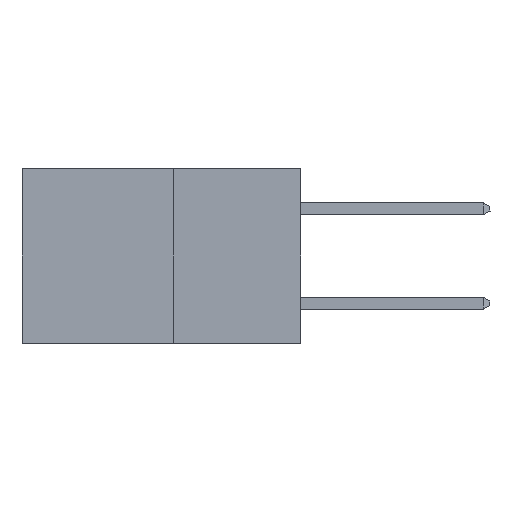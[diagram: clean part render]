
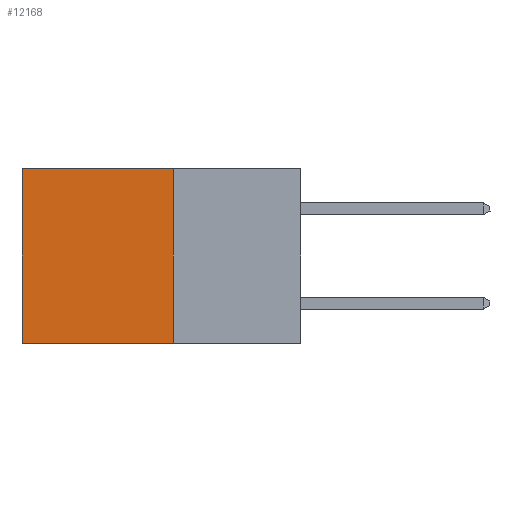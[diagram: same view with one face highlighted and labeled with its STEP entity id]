
A CAD part, left-side view. The second image highlights one B-rep face of the part: STEP entity #12168.
In plain terms, the highlighted planar face has unit normal (-1, 0, 0).
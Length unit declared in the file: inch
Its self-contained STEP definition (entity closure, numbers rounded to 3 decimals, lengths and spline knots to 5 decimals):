
#164 = VERTEX_POINT ( 'NONE', #13978 ) ;
#194 = DIRECTION ( 'NONE',  ( 1., 0., 0. ) ) ;
#1376 = ORIENTED_EDGE ( 'NONE', *, *, #3615, .F. ) ;
#1487 = CARTESIAN_POINT ( 'NONE',  ( 0.277, 0.27, -0.37 ) ) ;
#1488 = CARTESIAN_POINT ( 'NONE',  ( 0.277, 0.27, 0. ) ) ;
#1641 = CARTESIAN_POINT ( 'NONE',  ( 0.277, 0.59, 0. ) ) ;
#1744 = VECTOR ( 'NONE', #15545, 39.37008 ) ;
#1748 = VERTEX_POINT ( 'NONE', #1641 ) ;
#1946 = FACE_OUTER_BOUND ( 'NONE', #13151, .T. ) ;
#2682 = VERTEX_POINT ( 'NONE', #1488 ) ;
#2818 = VECTOR ( 'NONE', #9699, 39.37008 ) ;
#3500 = CARTESIAN_POINT ( 'NONE',  ( 0.277, 0.27, 0. ) ) ;
#3615 = EDGE_CURVE ( 'NONE', #6841, #164, #3767, .T. ) ;
#3767 = LINE ( 'NONE', #7344, #7003 ) ;
#3879 = LINE ( 'NONE', #17012, #10702 ) ;
#4131 = PLANE ( 'NONE',  #14023 ) ;
#4514 = ORIENTED_EDGE ( 'NONE', *, *, #10122, .F. ) ;
#5972 = CARTESIAN_POINT ( 'NONE',  ( 0.277, 0.27, -0.37 ) ) ;
#6841 = VERTEX_POINT ( 'NONE', #5972 ) ;
#6894 = LINE ( 'NONE', #13637, #2818 ) ;
#7003 = VECTOR ( 'NONE', #15319, 39.37008 ) ;
#7344 = CARTESIAN_POINT ( 'NONE',  ( 0.277, 0.27, -0.37 ) ) ;
#8014 = ORIENTED_EDGE ( 'NONE', *, *, #10437, .T. ) ;
#9694 = DIRECTION ( 'NONE',  ( 0., 0., -1. ) ) ;
#9699 = DIRECTION ( 'NONE',  ( 0., 0., -1. ) ) ;
#10122 = EDGE_CURVE ( 'NONE', #2682, #6841, #6894, .T. ) ;
#10437 = EDGE_CURVE ( 'NONE', #2682, #1748, #12525, .T. ) ;
#10702 = VECTOR ( 'NONE', #15786, 39.37008 ) ;
#11675 = ORIENTED_EDGE ( 'NONE', *, *, #16898, .T. ) ;
#12168 = ADVANCED_FACE ( 'NONE', ( #1946 ), #4131, .F. ) ;
#12525 = LINE ( 'NONE', #3500, #1744 ) ;
#13151 = EDGE_LOOP ( 'NONE', ( #11675, #1376, #4514, #8014 ) ) ;
#13637 = CARTESIAN_POINT ( 'NONE',  ( 0.277, 0.27, -0.37 ) ) ;
#13978 = CARTESIAN_POINT ( 'NONE',  ( 0.277, 0.59, -0.37 ) ) ;
#14023 = AXIS2_PLACEMENT_3D ( 'NONE', #1487, #194, #9694 ) ;
#15319 = DIRECTION ( 'NONE',  ( 0., 1., 0. ) ) ;
#15545 = DIRECTION ( 'NONE',  ( 0., 1., 0. ) ) ;
#15786 = DIRECTION ( 'NONE',  ( 0., 0., -1. ) ) ;
#16898 = EDGE_CURVE ( 'NONE', #1748, #164, #3879, .T. ) ;
#17012 = CARTESIAN_POINT ( 'NONE',  ( 0.277, 0.59, -0.37 ) ) ;
